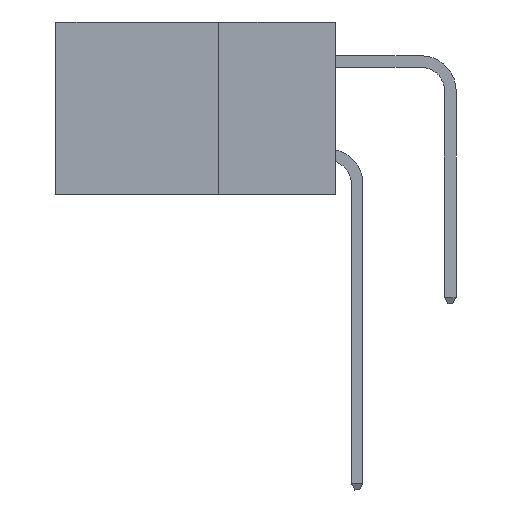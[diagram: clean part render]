
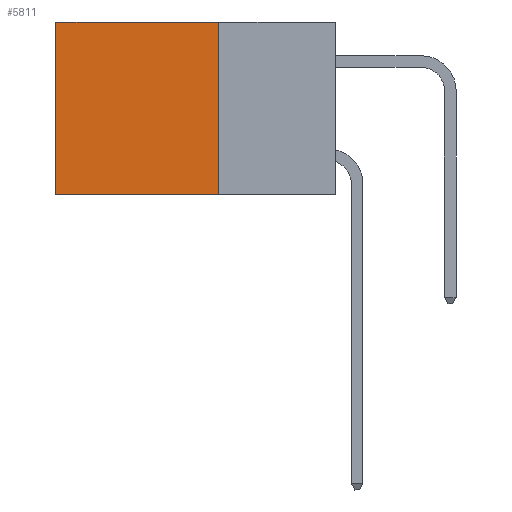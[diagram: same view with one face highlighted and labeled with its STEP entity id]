
A CAD part, left-side view. The second image highlights one B-rep face of the part: STEP entity #5811.
In plain terms, the highlighted planar face has unit normal (-1, 0, 0).
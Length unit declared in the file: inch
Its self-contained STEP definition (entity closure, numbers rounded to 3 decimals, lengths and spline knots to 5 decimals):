
#493 = CARTESIAN_POINT ( 'NONE',  ( 0.2875, 0.25, -0.37 ) ) ;
#622 = VECTOR ( 'NONE', #10168, 39.37008 ) ;
#1389 = LINE ( 'NONE', #2642, #8788 ) ;
#2476 = FACE_OUTER_BOUND ( 'NONE', #10287, .T. ) ;
#2642 = CARTESIAN_POINT ( 'NONE',  ( 0.2875, 0.25, 0. ) ) ;
#3393 = DIRECTION ( 'NONE',  ( 0., 1., 0. ) ) ;
#3586 = CARTESIAN_POINT ( 'NONE',  ( 0.2875, 0.6, -0.37 ) ) ;
#4006 = CARTESIAN_POINT ( 'NONE',  ( 0.2875, 0.25, 0. ) ) ;
#4156 = EDGE_CURVE ( 'NONE', #6291, #9471, #1389, .T. ) ;
#4559 = AXIS2_PLACEMENT_3D ( 'NONE', #10457, #6181, #8719 ) ;
#4843 = EDGE_CURVE ( 'NONE', #9471, #5201, #13526, .T. ) ;
#5201 = VERTEX_POINT ( 'NONE', #3586 ) ;
#5659 = CARTESIAN_POINT ( 'NONE',  ( 0.2875, 0.6, 0. ) ) ;
#5804 = CARTESIAN_POINT ( 'NONE',  ( 0.2875, 0.25, 0. ) ) ;
#5811 = ADVANCED_FACE ( 'NONE', ( #2476 ), #10401, .F. ) ;
#6181 = DIRECTION ( 'NONE',  ( 1., 0., 0. ) ) ;
#6291 = VERTEX_POINT ( 'NONE', #4006 ) ;
#6541 = ORIENTED_EDGE ( 'NONE', *, *, #4843, .F. ) ;
#7108 = LINE ( 'NONE', #5804, #8784 ) ;
#7411 = CARTESIAN_POINT ( 'NONE',  ( 0.2875, 0.6, 0. ) ) ;
#7570 = DIRECTION ( 'NONE',  ( 0., 0., -1. ) ) ;
#7708 = VECTOR ( 'NONE', #9642, 39.37008 ) ;
#7843 = ORIENTED_EDGE ( 'NONE', *, *, #10644, .T. ) ;
#8719 = DIRECTION ( 'NONE',  ( 0., 0., -1. ) ) ;
#8784 = VECTOR ( 'NONE', #3393, 39.37008 ) ;
#8788 = VECTOR ( 'NONE', #7570, 39.37008 ) ;
#8834 = LINE ( 'NONE', #7411, #7708 ) ;
#9471 = VERTEX_POINT ( 'NONE', #493 ) ;
#9642 = DIRECTION ( 'NONE',  ( 0., 0., -1. ) ) ;
#10168 = DIRECTION ( 'NONE',  ( 0., 1., 0. ) ) ;
#10287 = EDGE_LOOP ( 'NONE', ( #7843, #6541, #14298, #14200 ) ) ;
#10401 = PLANE ( 'NONE',  #4559 ) ;
#10457 = CARTESIAN_POINT ( 'NONE',  ( 0.2875, 0.25, 0. ) ) ;
#10644 = EDGE_CURVE ( 'NONE', #12596, #5201, #8834, .T. ) ;
#12596 = VERTEX_POINT ( 'NONE', #5659 ) ;
#12724 = CARTESIAN_POINT ( 'NONE',  ( 0.2875, 0.25, -0.37 ) ) ;
#12725 = EDGE_CURVE ( 'NONE', #6291, #12596, #7108, .T. ) ;
#13526 = LINE ( 'NONE', #12724, #622 ) ;
#14200 = ORIENTED_EDGE ( 'NONE', *, *, #12725, .T. ) ;
#14298 = ORIENTED_EDGE ( 'NONE', *, *, #4156, .F. ) ;
